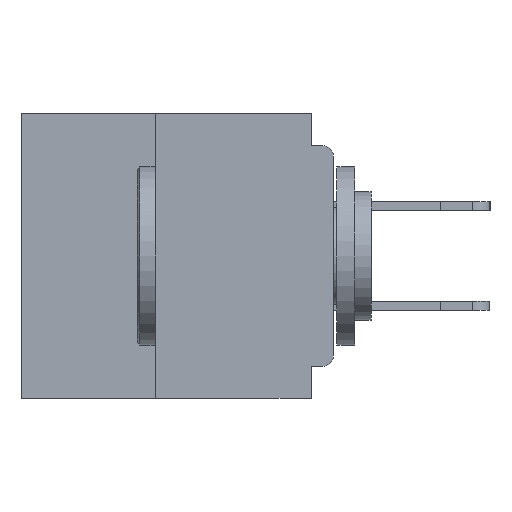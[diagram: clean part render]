
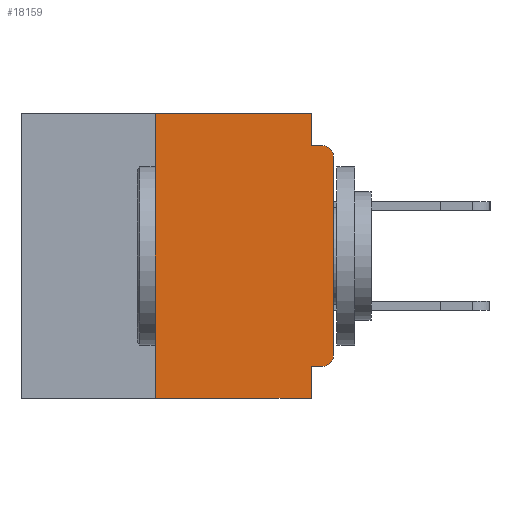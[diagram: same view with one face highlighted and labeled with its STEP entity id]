
A CAD part, left-side view. The second image highlights one B-rep face of the part: STEP entity #18159.
In plain terms, the highlighted planar face has unit normal (-1, 0, 0).
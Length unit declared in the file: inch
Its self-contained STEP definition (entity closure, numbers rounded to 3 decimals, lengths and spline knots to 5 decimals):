
#49 = VERTEX_POINT ( 'NONE', #3776 ) ;
#884 = DIRECTION ( 'NONE',  ( 1., 0., 0. ) ) ;
#1202 = CARTESIAN_POINT ( 'NONE',  ( 0., 0.25, -0.4 ) ) ;
#1224 = ORIENTED_EDGE ( 'NONE', *, *, #27893, .F. ) ;
#1473 = EDGE_CURVE ( 'NONE', #28959, #7132, #41462, .T. ) ;
#1967 = CARTESIAN_POINT ( 'NONE',  ( 0., 0., -0.06 ) ) ;
#3776 = CARTESIAN_POINT ( 'NONE',  ( 0., 0.015, -0.045 ) ) ;
#3984 = PLANE ( 'NONE',  #18545 ) ;
#4838 = CARTESIAN_POINT ( 'NONE',  ( 0., 0., -0.355 ) ) ;
#5018 = DIRECTION ( 'NONE',  ( 0., 0., 1. ) ) ;
#5509 = DIRECTION ( 'NONE',  ( -1., 0., 0. ) ) ;
#5628 = LINE ( 'NONE', #40736, #38246 ) ;
#5804 = DIRECTION ( 'NONE',  ( 0., -1., 0. ) ) ;
#6441 = LINE ( 'NONE', #31006, #39049 ) ;
#6476 = VERTEX_POINT ( 'NONE', #8226 ) ;
#6803 = ORIENTED_EDGE ( 'NONE', *, *, #34232, .F. ) ;
#7132 = VERTEX_POINT ( 'NONE', #38227 ) ;
#7504 = EDGE_CURVE ( 'NONE', #25106, #12122, #11615, .T. ) ;
#7820 = DIRECTION ( 'NONE',  ( 0., -1., 0. ) ) ;
#7977 = DIRECTION ( 'NONE',  ( 0., 0., -1. ) ) ;
#8108 = EDGE_LOOP ( 'NONE', ( #18091, #28761, #40439, #6803, #1224, #35887, #38913, #14018, #34383, #18131 ) ) ;
#8116 = DIRECTION ( 'NONE',  ( 0., 1., 0. ) ) ;
#8226 = CARTESIAN_POINT ( 'NONE',  ( 0., 0.031, 0. ) ) ;
#9592 = VERTEX_POINT ( 'NONE', #38872 ) ;
#10258 = LINE ( 'NONE', #25327, #15346 ) ;
#11054 = CARTESIAN_POINT ( 'NONE',  ( 0., 0.015, -0.355 ) ) ;
#11615 = LINE ( 'NONE', #4838, #27956 ) ;
#11675 = VERTEX_POINT ( 'NONE', #28717 ) ;
#12122 = VERTEX_POINT ( 'NONE', #31662 ) ;
#12713 = VERTEX_POINT ( 'NONE', #1967 ) ;
#13060 = LINE ( 'NONE', #24345, #29358 ) ;
#14018 = ORIENTED_EDGE ( 'NONE', *, *, #41578, .F. ) ;
#14620 = EDGE_CURVE ( 'NONE', #28959, #39791, #6441, .T. ) ;
#14768 = AXIS2_PLACEMENT_3D ( 'NONE', #16437, #39128, #19705 ) ;
#15346 = VECTOR ( 'NONE', #28614, 39.37008 ) ;
#16437 = CARTESIAN_POINT ( 'NONE',  ( 0., 0.015, -0.34 ) ) ;
#16963 = CARTESIAN_POINT ( 'NONE',  ( 0., 0.437, -0.4 ) ) ;
#17059 = LINE ( 'NONE', #30839, #23645 ) ;
#18091 = ORIENTED_EDGE ( 'NONE', *, *, #22052, .T. ) ;
#18131 = ORIENTED_EDGE ( 'NONE', *, *, #28028, .T. ) ;
#18159 = ADVANCED_FACE ( 'NONE', ( #36021 ), #3984, .F. ) ;
#18545 = AXIS2_PLACEMENT_3D ( 'NONE', #33374, #884, #23707 ) ;
#19705 = DIRECTION ( 'NONE',  ( 0., 0., -1. ) ) ;
#22052 = EDGE_CURVE ( 'NONE', #11675, #12713, #5628, .T. ) ;
#22124 = CARTESIAN_POINT ( 'NONE',  ( 0., 0.437, 0. ) ) ;
#22849 = EDGE_CURVE ( 'NONE', #9592, #49, #10258, .T. ) ;
#23645 = VECTOR ( 'NONE', #7977, 39.37008 ) ;
#23707 = DIRECTION ( 'NONE',  ( 0., 0., -1. ) ) ;
#24345 = CARTESIAN_POINT ( 'NONE',  ( 0., 0.031, -0.4 ) ) ;
#24544 = DIRECTION ( 'NONE',  ( 0., 0., 1. ) ) ;
#25036 = LINE ( 'NONE', #22124, #32667 ) ;
#25087 = CARTESIAN_POINT ( 'NONE',  ( 0., 0.015, -0.06 ) ) ;
#25106 = VERTEX_POINT ( 'NONE', #11054 ) ;
#25327 = CARTESIAN_POINT ( 'NONE',  ( 0., 0., -0.045 ) ) ;
#27578 = CIRCLE ( 'NONE', #14768, 0.015 ) ;
#27893 = EDGE_CURVE ( 'NONE', #39791, #6476, #25036, .T. ) ;
#27956 = VECTOR ( 'NONE', #8116, 39.37008 ) ;
#28028 = EDGE_CURVE ( 'NONE', #25106, #11675, #27578, .T. ) ;
#28376 = DIRECTION ( 'NONE',  ( 0., 0., -1. ) ) ;
#28614 = DIRECTION ( 'NONE',  ( 0., -1., 0. ) ) ;
#28717 = CARTESIAN_POINT ( 'NONE',  ( 0., 0., -0.34 ) ) ;
#28761 = ORIENTED_EDGE ( 'NONE', *, *, #41099, .T. ) ;
#28959 = VERTEX_POINT ( 'NONE', #1202 ) ;
#29358 = VECTOR ( 'NONE', #40533, 39.37008 ) ;
#30592 = CARTESIAN_POINT ( 'NONE',  ( 0., 0.25, 0. ) ) ;
#30839 = CARTESIAN_POINT ( 'NONE',  ( 0., 0.031, 0. ) ) ;
#31006 = CARTESIAN_POINT ( 'NONE',  ( 0., 0.25, -0.4 ) ) ;
#31662 = CARTESIAN_POINT ( 'NONE',  ( 0., 0.031, -0.355 ) ) ;
#32667 = VECTOR ( 'NONE', #5804, 39.37008 ) ;
#32810 = VECTOR ( 'NONE', #7820, 39.37008 ) ;
#33374 = CARTESIAN_POINT ( 'NONE',  ( 0., 0.437, 0. ) ) ;
#33810 = AXIS2_PLACEMENT_3D ( 'NONE', #25087, #5509, #28376 ) ;
#34232 = EDGE_CURVE ( 'NONE', #6476, #9592, #17059, .T. ) ;
#34383 = ORIENTED_EDGE ( 'NONE', *, *, #7504, .F. ) ;
#35887 = ORIENTED_EDGE ( 'NONE', *, *, #14620, .F. ) ;
#36021 = FACE_OUTER_BOUND ( 'NONE', #8108, .T. ) ;
#38227 = CARTESIAN_POINT ( 'NONE',  ( 0., 0.031, -0.4 ) ) ;
#38246 = VECTOR ( 'NONE', #24544, 39.37008 ) ;
#38872 = CARTESIAN_POINT ( 'NONE',  ( 0., 0.031, -0.045 ) ) ;
#38913 = ORIENTED_EDGE ( 'NONE', *, *, #1473, .T. ) ;
#39049 = VECTOR ( 'NONE', #5018, 39.37008 ) ;
#39128 = DIRECTION ( 'NONE',  ( -1., 0., 0. ) ) ;
#39791 = VERTEX_POINT ( 'NONE', #30592 ) ;
#40439 = ORIENTED_EDGE ( 'NONE', *, *, #22849, .F. ) ;
#40533 = DIRECTION ( 'NONE',  ( 0., 0., -1. ) ) ;
#40736 = CARTESIAN_POINT ( 'NONE',  ( 0., 0., 0. ) ) ;
#41093 = CIRCLE ( 'NONE', #33810, 0.015 ) ;
#41099 = EDGE_CURVE ( 'NONE', #12713, #49, #41093, .T. ) ;
#41462 = LINE ( 'NONE', #16963, #32810 ) ;
#41578 = EDGE_CURVE ( 'NONE', #12122, #7132, #13060, .T. ) ;
